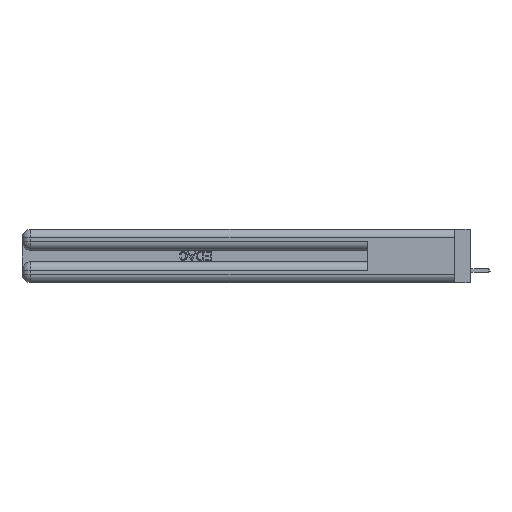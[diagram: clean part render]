
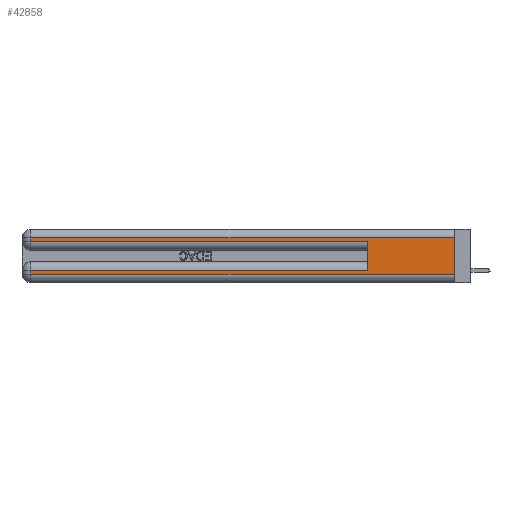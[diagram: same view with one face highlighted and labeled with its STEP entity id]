
A CAD part, left-side view. The second image highlights one B-rep face of the part: STEP entity #42858.
In plain terms, the highlighted planar face has unit normal (-1, 0, 0).
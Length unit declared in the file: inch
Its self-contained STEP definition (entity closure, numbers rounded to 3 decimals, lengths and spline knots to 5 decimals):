
#447 = VECTOR ( 'NONE', #1099, 39.37008 ) ;
#1099 = DIRECTION ( 'NONE',  ( 0., 0., 1. ) ) ;
#1561 = LINE ( 'NONE', #34220, #43473 ) ;
#1789 = CARTESIAN_POINT ( 'NONE',  ( 0., 0., 0.37 ) ) ;
#2228 = ORIENTED_EDGE ( 'NONE', *, *, #16671, .T. ) ;
#3124 = CARTESIAN_POINT ( 'NONE',  ( 0., 0., 0.285 ) ) ;
#4708 = CARTESIAN_POINT ( 'NONE',  ( 0., 2.94, 0.31 ) ) ;
#4868 = LINE ( 'NONE', #41400, #21700 ) ;
#6651 = CARTESIAN_POINT ( 'NONE',  ( 0., 0., 0.06 ) ) ;
#7550 = VERTEX_POINT ( 'NONE', #16467 ) ;
#8146 = VECTOR ( 'NONE', #17387, 39.37008 ) ;
#8984 = DIRECTION ( 'NONE',  ( 0., 0., -1. ) ) ;
#9547 = DIRECTION ( 'NONE',  ( 0., 0., -1. ) ) ;
#9651 = DIRECTION ( 'NONE',  ( 0., 1., 0. ) ) ;
#10165 = VERTEX_POINT ( 'NONE', #4708 ) ;
#10199 = CARTESIAN_POINT ( 'NONE',  ( 0., 2.94, 0.37 ) ) ;
#10333 = DIRECTION ( 'NONE',  ( 0., -1., 0. ) ) ;
#11825 = CARTESIAN_POINT ( 'NONE',  ( 0., 0.6, 0.285 ) ) ;
#12074 = DIRECTION ( 'NONE',  ( 0., 1., 0. ) ) ;
#12186 = EDGE_LOOP ( 'NONE', ( #26162, #39291, #41667, #33432, #35735, #38927, #2228, #24397 ) ) ;
#13849 = VERTEX_POINT ( 'NONE', #34164 ) ;
#14167 = VERTEX_POINT ( 'NONE', #44529 ) ;
#14643 = EDGE_CURVE ( 'NONE', #13849, #31923, #22262, .T. ) ;
#14756 = LINE ( 'NONE', #41223, #44407 ) ;
#15268 = CARTESIAN_POINT ( 'NONE',  ( 0., 0.6, 0.145 ) ) ;
#16467 = CARTESIAN_POINT ( 'NONE',  ( 0., 0., 0.31 ) ) ;
#16671 = EDGE_CURVE ( 'NONE', #14167, #31128, #21619, .T. ) ;
#16771 = LINE ( 'NONE', #20209, #40226 ) ;
#17387 = DIRECTION ( 'NONE',  ( 0., 0., -1. ) ) ;
#19434 = CARTESIAN_POINT ( 'NONE',  ( 0., 2.94, 0.06 ) ) ;
#20209 = CARTESIAN_POINT ( 'NONE',  ( 0., 0., 0.06 ) ) ;
#20250 = EDGE_CURVE ( 'NONE', #31128, #25811, #16771, .T. ) ;
#20837 = EDGE_CURVE ( 'NONE', #36922, #31923, #44380, .T. ) ;
#21619 = LINE ( 'NONE', #10199, #8146 ) ;
#21700 = VECTOR ( 'NONE', #9547, 39.37008 ) ;
#22262 = LINE ( 'NONE', #15268, #447 ) ;
#22274 = CARTESIAN_POINT ( 'NONE',  ( 0., 0., 0.31 ) ) ;
#22897 = PLANE ( 'NONE',  #29986 ) ;
#24397 = ORIENTED_EDGE ( 'NONE', *, *, #20250, .T. ) ;
#25006 = LINE ( 'NONE', #22274, #29403 ) ;
#25811 = VERTEX_POINT ( 'NONE', #6651 ) ;
#26162 = ORIENTED_EDGE ( 'NONE', *, *, #29690, .F. ) ;
#26871 = DIRECTION ( 'NONE',  ( 0., 0., -1. ) ) ;
#27637 = CARTESIAN_POINT ( 'NONE',  ( 0., 2.94, 0.285 ) ) ;
#29086 = EDGE_CURVE ( 'NONE', #13849, #14167, #1561, .T. ) ;
#29193 = FACE_OUTER_BOUND ( 'NONE', #12186, .T. ) ;
#29403 = VECTOR ( 'NONE', #12074, 39.37008 ) ;
#29690 = EDGE_CURVE ( 'NONE', #7550, #25811, #4868, .T. ) ;
#29707 = VECTOR ( 'NONE', #10333, 39.37008 ) ;
#29986 = AXIS2_PLACEMENT_3D ( 'NONE', #1789, #40535, #8984 ) ;
#31128 = VERTEX_POINT ( 'NONE', #19434 ) ;
#31639 = DIRECTION ( 'NONE',  ( 0., -1., 0. ) ) ;
#31923 = VERTEX_POINT ( 'NONE', #11825 ) ;
#33432 = ORIENTED_EDGE ( 'NONE', *, *, #20837, .T. ) ;
#34164 = CARTESIAN_POINT ( 'NONE',  ( 0., 0.6, 0.085 ) ) ;
#34220 = CARTESIAN_POINT ( 'NONE',  ( 0., 0., 0.085 ) ) ;
#35735 = ORIENTED_EDGE ( 'NONE', *, *, #14643, .F. ) ;
#36922 = VERTEX_POINT ( 'NONE', #27637 ) ;
#38927 = ORIENTED_EDGE ( 'NONE', *, *, #29086, .T. ) ;
#39182 = EDGE_CURVE ( 'NONE', #7550, #10165, #25006, .T. ) ;
#39291 = ORIENTED_EDGE ( 'NONE', *, *, #39182, .T. ) ;
#40226 = VECTOR ( 'NONE', #31639, 39.37008 ) ;
#40535 = DIRECTION ( 'NONE',  ( 1., 0., 0. ) ) ;
#41223 = CARTESIAN_POINT ( 'NONE',  ( 0., 2.94, 0.37 ) ) ;
#41378 = EDGE_CURVE ( 'NONE', #10165, #36922, #14756, .T. ) ;
#41400 = CARTESIAN_POINT ( 'NONE',  ( 0., 0., 0.37 ) ) ;
#41667 = ORIENTED_EDGE ( 'NONE', *, *, #41378, .T. ) ;
#42858 = ADVANCED_FACE ( 'NONE', ( #29193 ), #22897, .F. ) ;
#43473 = VECTOR ( 'NONE', #9651, 39.37008 ) ;
#44380 = LINE ( 'NONE', #3124, #29707 ) ;
#44407 = VECTOR ( 'NONE', #26871, 39.37008 ) ;
#44529 = CARTESIAN_POINT ( 'NONE',  ( 0., 2.94, 0.085 ) ) ;
